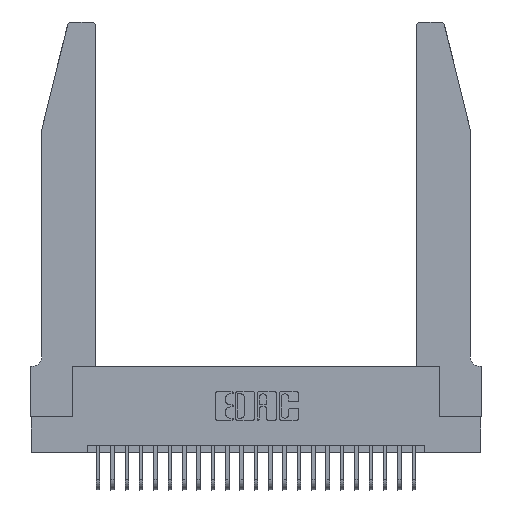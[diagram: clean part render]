
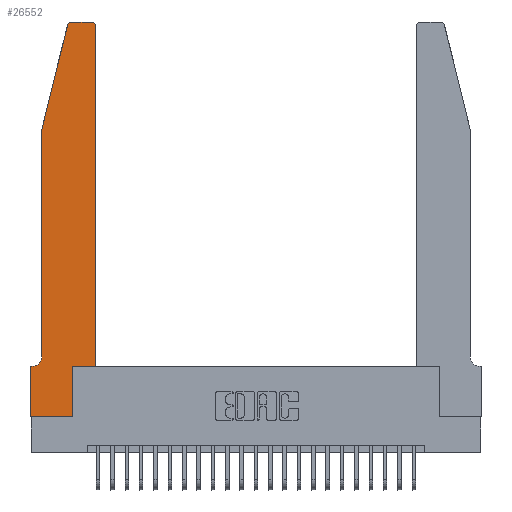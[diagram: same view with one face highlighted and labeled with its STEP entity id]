
A CAD part, top view. The second image highlights one B-rep face of the part: STEP entity #26552.
In plain terms, the highlighted planar face has unit normal (0, 0, 1).
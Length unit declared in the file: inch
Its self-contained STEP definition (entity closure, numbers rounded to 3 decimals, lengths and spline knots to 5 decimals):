
#807 = VERTEX_POINT ( 'NONE', #14983 ) ;
#816 = VECTOR ( 'NONE', #11751, 39.37008 ) ;
#1006 = VECTOR ( 'NONE', #10566, 39.37008 ) ;
#1059 = VECTOR ( 'NONE', #20007, 39.37008 ) ;
#1142 = DIRECTION ( 'NONE',  ( 0., 0., 1. ) ) ;
#1380 = LINE ( 'NONE', #20924, #6433 ) ;
#1722 = LINE ( 'NONE', #9034, #12456 ) ;
#2391 = ORIENTED_EDGE ( 'NONE', *, *, #19576, .T. ) ;
#2434 = ORIENTED_EDGE ( 'NONE', *, *, #2457, .T. ) ;
#2457 = EDGE_CURVE ( 'NONE', #24177, #807, #25283, .T. ) ;
#2526 = EDGE_CURVE ( 'NONE', #16395, #18041, #18783, .T. ) ;
#2935 = EDGE_LOOP ( 'NONE', ( #13812, #17040, #15304, #23956, #12321, #16679, #24406, #8728, #25070, #2391, #7263, #2434 ) ) ;
#3469 = VERTEX_POINT ( 'NONE', #22236 ) ;
#4009 = CARTESIAN_POINT ( 'NONE',  ( 0.25487, 2.72718, 0.37 ) ) ;
#4697 = DIRECTION ( 'NONE',  ( -1., 0., 0. ) ) ;
#4791 = CARTESIAN_POINT ( 'NONE',  ( 0.0755, 0.35, 0.37 ) ) ;
#4926 = DIRECTION ( 'NONE',  ( 1., 0., 0. ) ) ;
#5306 = VERTEX_POINT ( 'NONE', #9951 ) ;
#5848 = DIRECTION ( 'NONE',  ( 1., 0., 0. ) ) ;
#6433 = VECTOR ( 'NONE', #27029, 39.37008 ) ;
#6621 = PLANE ( 'NONE',  #11618 ) ;
#6733 = LINE ( 'NONE', #20810, #1006 ) ;
#6753 = VERTEX_POINT ( 'NONE', #23217 ) ;
#7263 = ORIENTED_EDGE ( 'NONE', *, *, #14256, .T. ) ;
#7582 = VECTOR ( 'NONE', #21473, 39.37008 ) ;
#8242 = AXIS2_PLACEMENT_3D ( 'NONE', #14739, #9527, #4926 ) ;
#8728 = ORIENTED_EDGE ( 'NONE', *, *, #13571, .T. ) ;
#8768 = CARTESIAN_POINT ( 'NONE',  ( 0., 0.35, 0.37 ) ) ;
#9034 = CARTESIAN_POINT ( 'NONE',  ( 0.2865, 0.35, 0.37 ) ) ;
#9134 = CARTESIAN_POINT ( 'NONE',  ( 0., 0., 0.37 ) ) ;
#9527 = DIRECTION ( 'NONE',  ( 0., 0., 1. ) ) ;
#9601 = CARTESIAN_POINT ( 'NONE',  ( 0.2605, 2.75, 0.37 ) ) ;
#9677 = DIRECTION ( 'NONE',  ( 1., 0., 0. ) ) ;
#9951 = CARTESIAN_POINT ( 'NONE',  ( 0.0755, 0.42, 0.37 ) ) ;
#10000 = VECTOR ( 'NONE', #14792, 39.37008 ) ;
#10192 = CARTESIAN_POINT ( 'NONE',  ( 0., 0., 0.37 ) ) ;
#10566 = DIRECTION ( 'NONE',  ( 0., -1., 0. ) ) ;
#10757 = AXIS2_PLACEMENT_3D ( 'NONE', #10843, #25158, #12970 ) ;
#10843 = CARTESIAN_POINT ( 'NONE',  ( 0.0055, 0.42, 0.37 ) ) ;
#10945 = DIRECTION ( 'NONE',  ( 0., 0., 1. ) ) ;
#10980 = CARTESIAN_POINT ( 'NONE',  ( 0.4505, 2.72, 0.37 ) ) ;
#11189 = LINE ( 'NONE', #10192, #16724 ) ;
#11353 = CARTESIAN_POINT ( 'NONE',  ( 0.284, 2.75, 0.37 ) ) ;
#11618 = AXIS2_PLACEMENT_3D ( 'NONE', #8768, #10945, #25259 ) ;
#11751 = DIRECTION ( 'NONE',  ( -1., 0., 0. ) ) ;
#12186 = EDGE_CURVE ( 'NONE', #6753, #18060, #15515, .T. ) ;
#12321 = ORIENTED_EDGE ( 'NONE', *, *, #16830, .T. ) ;
#12326 = EDGE_CURVE ( 'NONE', #807, #16395, #18359, .T. ) ;
#12456 = VECTOR ( 'NONE', #19388, 39.37008 ) ;
#12472 = LINE ( 'NONE', #17996, #1059 ) ;
#12605 = LINE ( 'NONE', #23451, #7582 ) ;
#12970 = DIRECTION ( 'NONE',  ( -1., 0., 0. ) ) ;
#13422 = CIRCLE ( 'NONE', #10757, 0.07 ) ;
#13571 = EDGE_CURVE ( 'NONE', #13873, #25900, #11189, .T. ) ;
#13812 = ORIENTED_EDGE ( 'NONE', *, *, #12326, .T. ) ;
#13873 = VERTEX_POINT ( 'NONE', #9134 ) ;
#14025 = EDGE_CURVE ( 'NONE', #18041, #3469, #12472, .T. ) ;
#14256 = EDGE_CURVE ( 'NONE', #21165, #24177, #1380, .T. ) ;
#14739 = CARTESIAN_POINT ( 'NONE',  ( 0.284, 2.72, 0.37 ) ) ;
#14792 = DIRECTION ( 'NONE',  ( 0., -1., 0. ) ) ;
#14931 = EDGE_CURVE ( 'NONE', #18060, #13873, #6733, .T. ) ;
#14983 = CARTESIAN_POINT ( 'NONE',  ( 0.4205, 2.75, 0.37 ) ) ;
#15304 = ORIENTED_EDGE ( 'NONE', *, *, #14025, .T. ) ;
#15515 = LINE ( 'NONE', #4791, #21495 ) ;
#15584 = LINE ( 'NONE', #22827, #10000 ) ;
#16395 = VERTEX_POINT ( 'NONE', #11353 ) ;
#16679 = ORIENTED_EDGE ( 'NONE', *, *, #12186, .T. ) ;
#16724 = VECTOR ( 'NONE', #5848, 39.37008 ) ;
#16830 = EDGE_CURVE ( 'NONE', #5306, #6753, #13422, .T. ) ;
#17040 = ORIENTED_EDGE ( 'NONE', *, *, #2526, .T. ) ;
#17996 = CARTESIAN_POINT ( 'NONE',  ( 0.0755, 2., 0.37 ) ) ;
#18041 = VERTEX_POINT ( 'NONE', #4009 ) ;
#18060 = VERTEX_POINT ( 'NONE', #22787 ) ;
#18359 = LINE ( 'NONE', #9601, #816 ) ;
#18783 = CIRCLE ( 'NONE', #8242, 0.03 ) ;
#19388 = DIRECTION ( 'NONE',  ( 0., 1., 0. ) ) ;
#19576 = EDGE_CURVE ( 'NONE', #24311, #21165, #12605, .T. ) ;
#19947 = AXIS2_PLACEMENT_3D ( 'NONE', #25119, #1142, #9677 ) ;
#19984 = CARTESIAN_POINT ( 'NONE',  ( 0.2865, 0.35, 0.37 ) ) ;
#20007 = DIRECTION ( 'NONE',  ( -0.239, -0.971, 0. ) ) ;
#20344 = FACE_OUTER_BOUND ( 'NONE', #2935, .T. ) ;
#20656 = CARTESIAN_POINT ( 'NONE',  ( 0.4505, 0.35, 0.37 ) ) ;
#20810 = CARTESIAN_POINT ( 'NONE',  ( 0., 0., 0.37 ) ) ;
#20924 = CARTESIAN_POINT ( 'NONE',  ( 0.4505, 0.35, 0.37 ) ) ;
#21165 = VERTEX_POINT ( 'NONE', #20656 ) ;
#21473 = DIRECTION ( 'NONE',  ( 1., 0., 0. ) ) ;
#21495 = VECTOR ( 'NONE', #4697, 39.37008 ) ;
#22236 = CARTESIAN_POINT ( 'NONE',  ( 0.0755, 2., 0.37 ) ) ;
#22710 = CARTESIAN_POINT ( 'NONE',  ( 0.2865, 0., 0.37 ) ) ;
#22787 = CARTESIAN_POINT ( 'NONE',  ( 0., 0.35, 0.37 ) ) ;
#22827 = CARTESIAN_POINT ( 'NONE',  ( 0.0755, 2., 0.37 ) ) ;
#23217 = CARTESIAN_POINT ( 'NONE',  ( 0.0055, 0.35, 0.37 ) ) ;
#23451 = CARTESIAN_POINT ( 'NONE',  ( 0.4505, 0.35, 0.37 ) ) ;
#23631 = EDGE_CURVE ( 'NONE', #25900, #24311, #1722, .T. ) ;
#23956 = ORIENTED_EDGE ( 'NONE', *, *, #26959, .T. ) ;
#24177 = VERTEX_POINT ( 'NONE', #10980 ) ;
#24311 = VERTEX_POINT ( 'NONE', #19984 ) ;
#24406 = ORIENTED_EDGE ( 'NONE', *, *, #14931, .T. ) ;
#25070 = ORIENTED_EDGE ( 'NONE', *, *, #23631, .T. ) ;
#25119 = CARTESIAN_POINT ( 'NONE',  ( 0.4205, 2.72, 0.37 ) ) ;
#25158 = DIRECTION ( 'NONE',  ( 0., 0., -1. ) ) ;
#25259 = DIRECTION ( 'NONE',  ( 1., 0., 0. ) ) ;
#25283 = CIRCLE ( 'NONE', #19947, 0.03 ) ;
#25900 = VERTEX_POINT ( 'NONE', #22710 ) ;
#26552 = ADVANCED_FACE ( 'NONE', ( #20344 ), #6621, .T. ) ;
#26959 = EDGE_CURVE ( 'NONE', #3469, #5306, #15584, .T. ) ;
#27029 = DIRECTION ( 'NONE',  ( 0., 1., 0. ) ) ;
